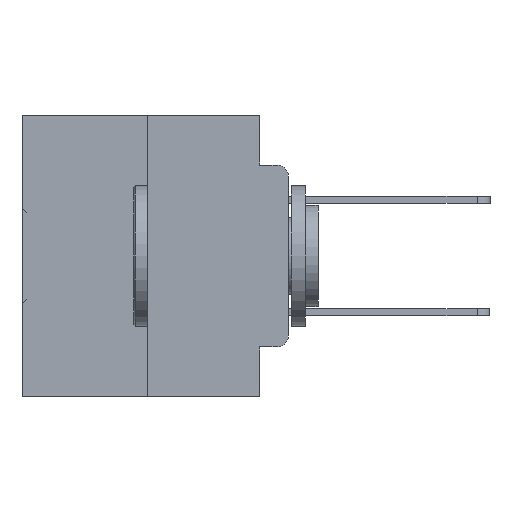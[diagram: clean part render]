
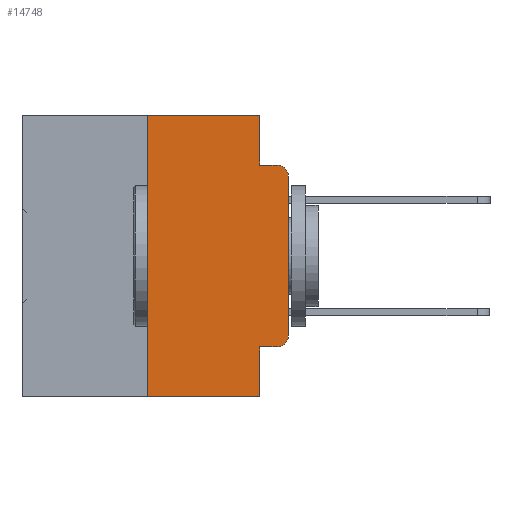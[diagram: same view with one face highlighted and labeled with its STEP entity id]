
A CAD part, left-side view. The second image highlights one B-rep face of the part: STEP entity #14748.
In plain terms, the highlighted planar face has unit normal (-1, 0, 0).
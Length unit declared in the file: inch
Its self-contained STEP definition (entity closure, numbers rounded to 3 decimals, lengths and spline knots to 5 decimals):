
#29 = CARTESIAN_POINT ( 'NONE',  ( 0., 0.051, -0.4115 ) ) ;
#100 = VECTOR ( 'NONE', #794, 39.37008 ) ;
#632 = LINE ( 'NONE', #8001, #7126 ) ;
#781 = CARTESIAN_POINT ( 'NONE',  ( 0., 0.25, 0. ) ) ;
#794 = DIRECTION ( 'NONE',  ( 0., -1., 0. ) ) ;
#878 = LINE ( 'NONE', #15883, #14611 ) ;
#954 = VERTEX_POINT ( 'NONE', #14164 ) ;
#1276 = VERTEX_POINT ( 'NONE', #17819 ) ;
#1941 = DIRECTION ( 'NONE',  ( 0., 0., -1. ) ) ;
#2201 = ORIENTED_EDGE ( 'NONE', *, *, #27225, .T. ) ;
#2396 = VERTEX_POINT ( 'NONE', #23798 ) ;
#2668 = VERTEX_POINT ( 'NONE', #8592 ) ;
#3437 = CARTESIAN_POINT ( 'NONE',  ( 0., 0., 0. ) ) ;
#4248 = AXIS2_PLACEMENT_3D ( 'NONE', #5724, #24470, #8536 ) ;
#4901 = VERTEX_POINT ( 'NONE', #25672 ) ;
#4956 = VECTOR ( 'NONE', #15558, 39.37008 ) ;
#5076 = ORIENTED_EDGE ( 'NONE', *, *, #11709, .F. ) ;
#5724 = CARTESIAN_POINT ( 'NONE',  ( 0., 0.02, -0.1085 ) ) ;
#5795 = CARTESIAN_POINT ( 'NONE',  ( 0., 0.051, 0. ) ) ;
#6602 = ORIENTED_EDGE ( 'NONE', *, *, #14340, .F. ) ;
#7126 = VECTOR ( 'NONE', #29385, 39.37008 ) ;
#7200 = EDGE_CURVE ( 'NONE', #33549, #17025, #25025, .T. ) ;
#7330 = VERTEX_POINT ( 'NONE', #20039 ) ;
#8001 = CARTESIAN_POINT ( 'NONE',  ( 0., 0.051, -0.0885 ) ) ;
#8285 = CARTESIAN_POINT ( 'NONE',  ( 0., 0.473, 0. ) ) ;
#8536 = DIRECTION ( 'NONE',  ( 0., 0., -1. ) ) ;
#8592 = CARTESIAN_POINT ( 'NONE',  ( 0., 0.051, -0.5 ) ) ;
#8607 = DIRECTION ( 'NONE',  ( 0., 0., -1. ) ) ;
#8685 = ORIENTED_EDGE ( 'NONE', *, *, #16571, .T. ) ;
#9086 = CARTESIAN_POINT ( 'NONE',  ( 0., 0.051, -0.4115 ) ) ;
#10161 = CARTESIAN_POINT ( 'NONE',  ( 0., 0.473, 0. ) ) ;
#11011 = PLANE ( 'NONE',  #17416 ) ;
#11155 = DIRECTION ( 'NONE',  ( 0., -1., 0. ) ) ;
#11709 = EDGE_CURVE ( 'NONE', #2396, #7330, #26348, .T. ) ;
#13141 = VECTOR ( 'NONE', #30274, 39.37008 ) ;
#14164 = CARTESIAN_POINT ( 'NONE',  ( 0., 0.051, -0.0885 ) ) ;
#14340 = EDGE_CURVE ( 'NONE', #31188, #2396, #27262, .T. ) ;
#14611 = VECTOR ( 'NONE', #18415, 39.37008 ) ;
#14748 = ADVANCED_FACE ( 'NONE', ( #21749 ), #11011, .F. ) ;
#15018 = ORIENTED_EDGE ( 'NONE', *, *, #33277, .F. ) ;
#15453 = EDGE_CURVE ( 'NONE', #7330, #954, #19651, .T. ) ;
#15558 = DIRECTION ( 'NONE',  ( 0., -1., 0. ) ) ;
#15883 = CARTESIAN_POINT ( 'NONE',  ( 0., 0.051, 0. ) ) ;
#16387 = DIRECTION ( 'NONE',  ( 0., 0., -1. ) ) ;
#16571 = EDGE_CURVE ( 'NONE', #1276, #4901, #25383, .T. ) ;
#17025 = VERTEX_POINT ( 'NONE', #18541 ) ;
#17108 = CARTESIAN_POINT ( 'NONE',  ( 0., 0.473, -0.5 ) ) ;
#17147 = VECTOR ( 'NONE', #11155, 39.37008 ) ;
#17416 = AXIS2_PLACEMENT_3D ( 'NONE', #8285, #32349, #16387 ) ;
#17819 = CARTESIAN_POINT ( 'NONE',  ( 0., 0., -0.1085 ) ) ;
#18233 = DIRECTION ( 'NONE',  ( -1., 0., 0. ) ) ;
#18415 = DIRECTION ( 'NONE',  ( 0., 0., -1. ) ) ;
#18541 = CARTESIAN_POINT ( 'NONE',  ( 0., 0.02, -0.4115 ) ) ;
#19651 = LINE ( 'NONE', #5795, #33045 ) ;
#20039 = CARTESIAN_POINT ( 'NONE',  ( 0., 0.051, 0. ) ) ;
#20640 = EDGE_CURVE ( 'NONE', #31188, #2668, #27980, .T. ) ;
#20657 = LINE ( 'NONE', #3437, #33235 ) ;
#21316 = CIRCLE ( 'NONE', #22534, 0.02 ) ;
#21485 = ORIENTED_EDGE ( 'NONE', *, *, #20640, .T. ) ;
#21749 = FACE_OUTER_BOUND ( 'NONE', #26714, .T. ) ;
#22534 = AXIS2_PLACEMENT_3D ( 'NONE', #34179, #18233, #1941 ) ;
#23661 = ORIENTED_EDGE ( 'NONE', *, *, #15453, .F. ) ;
#23798 = CARTESIAN_POINT ( 'NONE',  ( 0., 0.25, 0. ) ) ;
#23812 = CARTESIAN_POINT ( 'NONE',  ( 0., 0., -0.3915 ) ) ;
#24470 = DIRECTION ( 'NONE',  ( -1., 0., 0. ) ) ;
#25025 = LINE ( 'NONE', #29, #17147 ) ;
#25107 = EDGE_CURVE ( 'NONE', #33549, #2668, #878, .T. ) ;
#25131 = VERTEX_POINT ( 'NONE', #23812 ) ;
#25383 = CIRCLE ( 'NONE', #4248, 0.02 ) ;
#25672 = CARTESIAN_POINT ( 'NONE',  ( 0., 0.02, -0.0885 ) ) ;
#26348 = LINE ( 'NONE', #10161, #4956 ) ;
#26714 = EDGE_LOOP ( 'NONE', ( #2201, #8685, #15018, #23661, #5076, #6602, #21485, #34874, #28573, #28167 ) ) ;
#27225 = EDGE_CURVE ( 'NONE', #25131, #1276, #20657, .T. ) ;
#27262 = LINE ( 'NONE', #781, #13141 ) ;
#27700 = DIRECTION ( 'NONE',  ( 0., 0., 1. ) ) ;
#27980 = LINE ( 'NONE', #17108, #100 ) ;
#28167 = ORIENTED_EDGE ( 'NONE', *, *, #29410, .T. ) ;
#28573 = ORIENTED_EDGE ( 'NONE', *, *, #7200, .T. ) ;
#29385 = DIRECTION ( 'NONE',  ( 0., -1., 0. ) ) ;
#29410 = EDGE_CURVE ( 'NONE', #17025, #25131, #21316, .T. ) ;
#30274 = DIRECTION ( 'NONE',  ( 0., 0., 1. ) ) ;
#30684 = CARTESIAN_POINT ( 'NONE',  ( 0., 0.25, -0.5 ) ) ;
#31188 = VERTEX_POINT ( 'NONE', #30684 ) ;
#32349 = DIRECTION ( 'NONE',  ( 1., 0., 0. ) ) ;
#33045 = VECTOR ( 'NONE', #8607, 39.37008 ) ;
#33235 = VECTOR ( 'NONE', #27700, 39.37008 ) ;
#33277 = EDGE_CURVE ( 'NONE', #954, #4901, #632, .T. ) ;
#33549 = VERTEX_POINT ( 'NONE', #9086 ) ;
#34179 = CARTESIAN_POINT ( 'NONE',  ( 0., 0.02, -0.3915 ) ) ;
#34874 = ORIENTED_EDGE ( 'NONE', *, *, #25107, .F. ) ;
